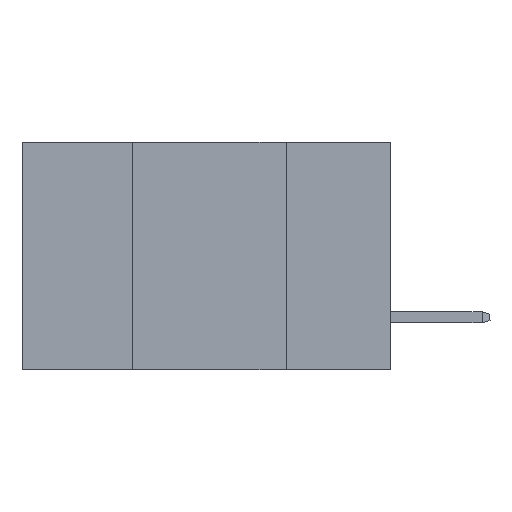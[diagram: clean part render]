
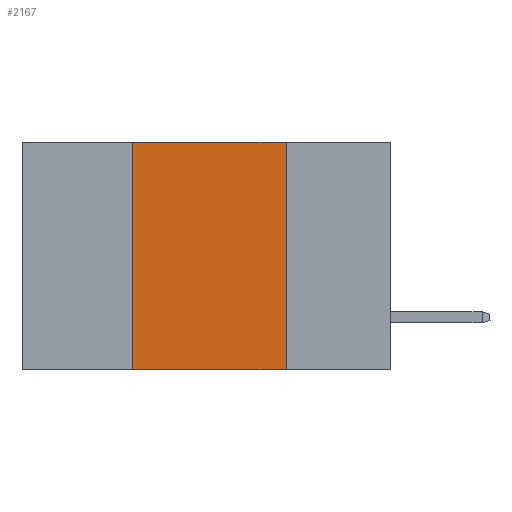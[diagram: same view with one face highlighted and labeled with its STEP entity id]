
A CAD part, left-side view. The second image highlights one B-rep face of the part: STEP entity #2167.
In plain terms, the highlighted planar face has unit normal (-1, 0, 0).
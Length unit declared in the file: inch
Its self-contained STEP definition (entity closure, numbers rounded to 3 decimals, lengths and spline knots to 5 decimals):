
#330 = VECTOR ( 'NONE', #5066, 39.37008 ) ;
#924 = PLANE ( 'NONE',  #1038 ) ;
#1038 = AXIS2_PLACEMENT_3D ( 'NONE', #17365, #13811, #2814 ) ;
#1135 = DIRECTION ( 'NONE',  ( 0., -1., 0. ) ) ;
#2167 = ADVANCED_FACE ( 'NONE', ( #13114 ), #924, .F. ) ;
#2484 = VERTEX_POINT ( 'NONE', #14673 ) ;
#2814 = DIRECTION ( 'NONE',  ( 0., 0., -1. ) ) ;
#3165 = LINE ( 'NONE', #12184, #16044 ) ;
#3245 = CARTESIAN_POINT ( 'NONE',  ( 0., 0.6, 0. ) ) ;
#3647 = EDGE_CURVE ( 'NONE', #22351, #6415, #11334, .T. ) ;
#3777 = VECTOR ( 'NONE', #21509, 39.37008 ) ;
#4544 = ORIENTED_EDGE ( 'NONE', *, *, #20442, .T. ) ;
#5066 = DIRECTION ( 'NONE',  ( 0., 0., 1. ) ) ;
#6240 = VERTEX_POINT ( 'NONE', #6347 ) ;
#6347 = CARTESIAN_POINT ( 'NONE',  ( 0., 0.17, 0. ) ) ;
#6415 = VERTEX_POINT ( 'NONE', #16045 ) ;
#7647 = CARTESIAN_POINT ( 'NONE',  ( 0., 0.17, 0. ) ) ;
#8591 = EDGE_CURVE ( 'NONE', #6240, #2484, #18026, .T. ) ;
#8995 = EDGE_CURVE ( 'NONE', #6415, #6240, #23137, .T. ) ;
#11147 = EDGE_LOOP ( 'NONE', ( #20995, #20328, #16897, #4544 ) ) ;
#11334 = LINE ( 'NONE', #12393, #330 ) ;
#12184 = CARTESIAN_POINT ( 'NONE',  ( 0., 0.6, -0.37 ) ) ;
#12307 = CARTESIAN_POINT ( 'NONE',  ( 0., 0.42, -0.37 ) ) ;
#12393 = CARTESIAN_POINT ( 'NONE',  ( 0., 0.42, 0. ) ) ;
#13114 = FACE_OUTER_BOUND ( 'NONE', #11147, .T. ) ;
#13811 = DIRECTION ( 'NONE',  ( 1., 0., 0. ) ) ;
#14673 = CARTESIAN_POINT ( 'NONE',  ( 0., 0.17, -0.37 ) ) ;
#16044 = VECTOR ( 'NONE', #1135, 39.37008 ) ;
#16045 = CARTESIAN_POINT ( 'NONE',  ( 0., 0.42, 0. ) ) ;
#16897 = ORIENTED_EDGE ( 'NONE', *, *, #3647, .F. ) ;
#17365 = CARTESIAN_POINT ( 'NONE',  ( 0., 0.6, 0. ) ) ;
#18026 = LINE ( 'NONE', #7647, #18599 ) ;
#18599 = VECTOR ( 'NONE', #20338, 39.37008 ) ;
#20328 = ORIENTED_EDGE ( 'NONE', *, *, #8995, .F. ) ;
#20338 = DIRECTION ( 'NONE',  ( 0., 0., -1. ) ) ;
#20442 = EDGE_CURVE ( 'NONE', #22351, #2484, #3165, .T. ) ;
#20995 = ORIENTED_EDGE ( 'NONE', *, *, #8591, .F. ) ;
#21509 = DIRECTION ( 'NONE',  ( 0., -1., 0. ) ) ;
#22351 = VERTEX_POINT ( 'NONE', #12307 ) ;
#23137 = LINE ( 'NONE', #3245, #3777 ) ;
